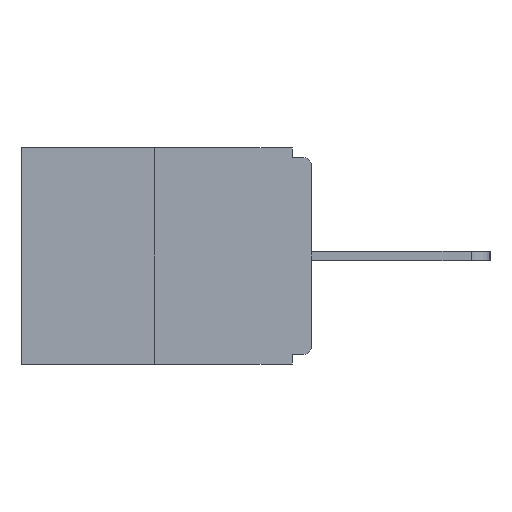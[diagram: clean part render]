
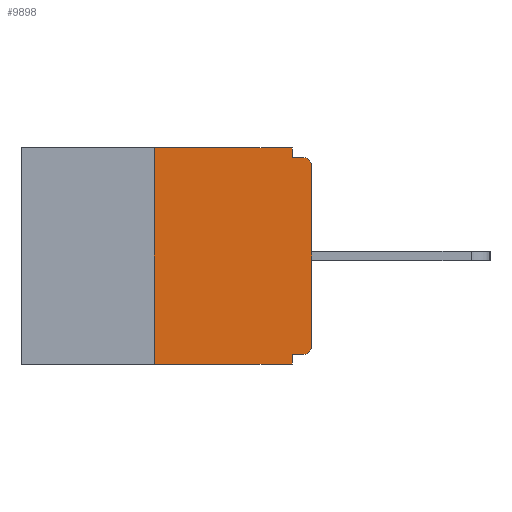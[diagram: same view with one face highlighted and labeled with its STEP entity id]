
A CAD part, left-side view. The second image highlights one B-rep face of the part: STEP entity #9898.
In plain terms, the highlighted planar face has unit normal (-1, 0, 0).
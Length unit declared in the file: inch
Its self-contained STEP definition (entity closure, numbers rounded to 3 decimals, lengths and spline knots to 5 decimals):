
#130 = CARTESIAN_POINT ( 'NONE',  ( 0., 0.031, 0. ) ) ;
#425 = DIRECTION ( 'NONE',  ( 0., 0., -1. ) ) ;
#506 = VECTOR ( 'NONE', #17227, 39.37008 ) ;
#839 = VERTEX_POINT ( 'NONE', #17845 ) ;
#925 = EDGE_CURVE ( 'NONE', #7638, #15540, #8388, .T. ) ;
#1435 = AXIS2_PLACEMENT_3D ( 'NONE', #9218, #16564, #425 ) ;
#1529 = VERTEX_POINT ( 'NONE', #1725 ) ;
#1725 = CARTESIAN_POINT ( 'NONE',  ( 0., 0.031, -0.015 ) ) ;
#1782 = ORIENTED_EDGE ( 'NONE', *, *, #11390, .F. ) ;
#1830 = FACE_OUTER_BOUND ( 'NONE', #5790, .T. ) ;
#1975 = ORIENTED_EDGE ( 'NONE', *, *, #13544, .F. ) ;
#2435 = VERTEX_POINT ( 'NONE', #3321 ) ;
#2648 = CIRCLE ( 'NONE', #1435, 0.015 ) ;
#2798 = DIRECTION ( 'NONE',  ( 0., -1., 0. ) ) ;
#3321 = CARTESIAN_POINT ( 'NONE',  ( 0., 0.015, -0.015 ) ) ;
#3402 = CARTESIAN_POINT ( 'NONE',  ( 0., 0.015, -0.313 ) ) ;
#3625 = DIRECTION ( 'NONE',  ( 0., -1., 0. ) ) ;
#3746 = VECTOR ( 'NONE', #12777, 39.37008 ) ;
#3762 = ORIENTED_EDGE ( 'NONE', *, *, #925, .T. ) ;
#3865 = VECTOR ( 'NONE', #7387, 39.37008 ) ;
#4063 = ORIENTED_EDGE ( 'NONE', *, *, #7671, .T. ) ;
#4079 = CARTESIAN_POINT ( 'NONE',  ( 0., 0., 0. ) ) ;
#4408 = LINE ( 'NONE', #15990, #18368 ) ;
#5740 = ORIENTED_EDGE ( 'NONE', *, *, #9665, .F. ) ;
#5790 = EDGE_LOOP ( 'NONE', ( #5740, #17530, #6524, #1782, #13985, #4063, #3762, #9715, #1975, #12144 ) ) ;
#6524 = ORIENTED_EDGE ( 'NONE', *, *, #9185, .T. ) ;
#6607 = CIRCLE ( 'NONE', #18183, 0.015 ) ;
#6746 = EDGE_CURVE ( 'NONE', #15540, #2435, #2648, .T. ) ;
#7031 = VECTOR ( 'NONE', #15267, 39.37008 ) ;
#7154 = EDGE_CURVE ( 'NONE', #16965, #14916, #17225, .T. ) ;
#7179 = VERTEX_POINT ( 'NONE', #11298 ) ;
#7387 = DIRECTION ( 'NONE',  ( 0., 1., 0. ) ) ;
#7638 = VERTEX_POINT ( 'NONE', #13829 ) ;
#7671 = EDGE_CURVE ( 'NONE', #16965, #7638, #6607, .T. ) ;
#7685 = PLANE ( 'NONE',  #18869 ) ;
#7725 = DIRECTION ( 'NONE',  ( 0., 0., -1. ) ) ;
#7734 = CARTESIAN_POINT ( 'NONE',  ( 0., 0.031, -0.343 ) ) ;
#8217 = LINE ( 'NONE', #8302, #18843 ) ;
#8302 = CARTESIAN_POINT ( 'NONE',  ( 0., 0.46, -0.343 ) ) ;
#8368 = VERTEX_POINT ( 'NONE', #130 ) ;
#8388 = LINE ( 'NONE', #4079, #3746 ) ;
#8481 = EDGE_CURVE ( 'NONE', #7179, #839, #8547, .T. ) ;
#8547 = LINE ( 'NONE', #11677, #506 ) ;
#8638 = CARTESIAN_POINT ( 'NONE',  ( 0., 0., -0.328 ) ) ;
#8922 = LINE ( 'NONE', #14738, #10922 ) ;
#9185 = EDGE_CURVE ( 'NONE', #7179, #12500, #8217, .T. ) ;
#9204 = DIRECTION ( 'NONE',  ( 0., 0., -1. ) ) ;
#9218 = CARTESIAN_POINT ( 'NONE',  ( 0., 0.015, -0.03 ) ) ;
#9665 = EDGE_CURVE ( 'NONE', #839, #8368, #8922, .T. ) ;
#9715 = ORIENTED_EDGE ( 'NONE', *, *, #6746, .T. ) ;
#9898 = ADVANCED_FACE ( 'NONE', ( #1830 ), #7685, .F. ) ;
#10816 = CARTESIAN_POINT ( 'NONE',  ( 0., 0.46, 0. ) ) ;
#10870 = LINE ( 'NONE', #7734, #7031 ) ;
#10922 = VECTOR ( 'NONE', #15913, 39.37008 ) ;
#11298 = CARTESIAN_POINT ( 'NONE',  ( 0., 0.25, -0.343 ) ) ;
#11390 = EDGE_CURVE ( 'NONE', #14916, #12500, #10870, .T. ) ;
#11677 = CARTESIAN_POINT ( 'NONE',  ( 0., 0.25, 0. ) ) ;
#12007 = CARTESIAN_POINT ( 'NONE',  ( 0., 0., -0.03 ) ) ;
#12144 = ORIENTED_EDGE ( 'NONE', *, *, #18049, .F. ) ;
#12500 = VERTEX_POINT ( 'NONE', #16535 ) ;
#12777 = DIRECTION ( 'NONE',  ( 0., 0., 1. ) ) ;
#13544 = EDGE_CURVE ( 'NONE', #1529, #2435, #4408, .T. ) ;
#13829 = CARTESIAN_POINT ( 'NONE',  ( 0., 0., -0.313 ) ) ;
#13985 = ORIENTED_EDGE ( 'NONE', *, *, #7154, .F. ) ;
#14494 = VECTOR ( 'NONE', #14623, 39.37008 ) ;
#14529 = LINE ( 'NONE', #17303, #14494 ) ;
#14623 = DIRECTION ( 'NONE',  ( 0., 0., -1. ) ) ;
#14738 = CARTESIAN_POINT ( 'NONE',  ( 0., 0.46, 0. ) ) ;
#14916 = VERTEX_POINT ( 'NONE', #18074 ) ;
#15267 = DIRECTION ( 'NONE',  ( 0., 0., -1. ) ) ;
#15377 = CARTESIAN_POINT ( 'NONE',  ( 0., 0.015, -0.328 ) ) ;
#15540 = VERTEX_POINT ( 'NONE', #12007 ) ;
#15913 = DIRECTION ( 'NONE',  ( 0., -1., 0. ) ) ;
#15990 = CARTESIAN_POINT ( 'NONE',  ( 0., 0., -0.015 ) ) ;
#16465 = DIRECTION ( 'NONE',  ( 1., 0., 0. ) ) ;
#16535 = CARTESIAN_POINT ( 'NONE',  ( 0., 0.031, -0.343 ) ) ;
#16564 = DIRECTION ( 'NONE',  ( -1., 0., 0. ) ) ;
#16965 = VERTEX_POINT ( 'NONE', #15377 ) ;
#17225 = LINE ( 'NONE', #8638, #3865 ) ;
#17227 = DIRECTION ( 'NONE',  ( 0., 0., 1. ) ) ;
#17303 = CARTESIAN_POINT ( 'NONE',  ( 0., 0.031, 0. ) ) ;
#17530 = ORIENTED_EDGE ( 'NONE', *, *, #8481, .F. ) ;
#17845 = CARTESIAN_POINT ( 'NONE',  ( 0., 0.25, 0. ) ) ;
#17925 = DIRECTION ( 'NONE',  ( -1., 0., 0. ) ) ;
#18049 = EDGE_CURVE ( 'NONE', #8368, #1529, #14529, .T. ) ;
#18074 = CARTESIAN_POINT ( 'NONE',  ( 0., 0.031, -0.328 ) ) ;
#18183 = AXIS2_PLACEMENT_3D ( 'NONE', #3402, #17925, #7725 ) ;
#18368 = VECTOR ( 'NONE', #2798, 39.37008 ) ;
#18843 = VECTOR ( 'NONE', #3625, 39.37008 ) ;
#18869 = AXIS2_PLACEMENT_3D ( 'NONE', #10816, #16465, #9204 ) ;
